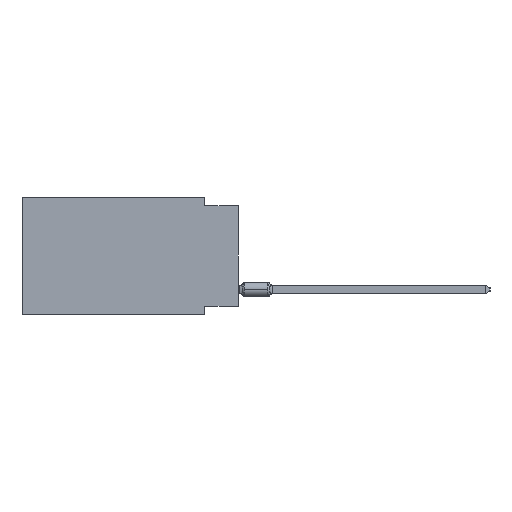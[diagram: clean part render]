
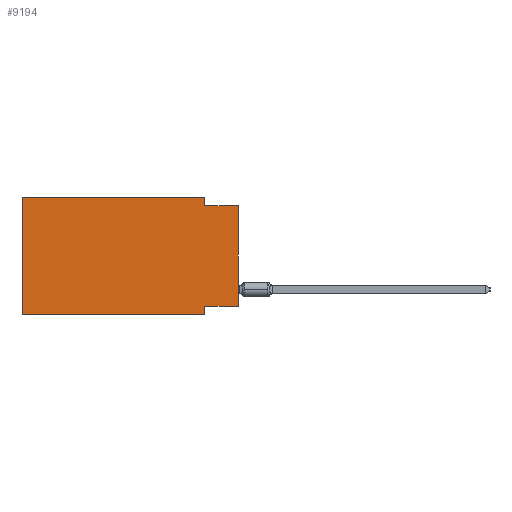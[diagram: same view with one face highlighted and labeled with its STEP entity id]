
A CAD part, left-side view. The second image highlights one B-rep face of the part: STEP entity #9194.
In plain terms, the highlighted planar face has unit normal (-1, 0, 0).
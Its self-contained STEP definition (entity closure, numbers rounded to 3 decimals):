
#537 = VECTOR ( 'NONE', #51391, 1000. ) ;
#1285 = VERTEX_POINT ( 'NONE', #85325 ) ;
#2928 = CARTESIAN_POINT ( 'NONE',  ( 0., 0., -8.255 ) ) ;
#6859 = AXIS2_PLACEMENT_3D ( 'NONE', #94778, #87290, #53614 ) ;
#9181 = ORIENTED_EDGE ( 'NONE', *, *, #14016, .T. ) ;
#9194 = ADVANCED_FACE ( 'NONE', ( #70192 ), #13004, .F. ) ;
#10488 = ORIENTED_EDGE ( 'NONE', *, *, #67953, .F. ) ;
#12084 = EDGE_CURVE ( 'NONE', #79813, #86254, #32679, .T. ) ;
#13004 = PLANE ( 'NONE',  #6859 ) ;
#14016 = EDGE_CURVE ( 'NONE', #24694, #28024, #19779, .T. ) ;
#16752 = EDGE_CURVE ( 'NONE', #86254, #28024, #59409, .T. ) ;
#16832 = EDGE_CURVE ( 'NONE', #98112, #1285, #22330, .T. ) ;
#16952 = EDGE_LOOP ( 'NONE', ( #55615, #24798, #31370, #48739, #10488, #9181, #80928, #34785 ) ) ;
#19779 = LINE ( 'NONE', #93534, #32743 ) ;
#20227 = LINE ( 'NONE', #103587, #83513 ) ;
#20298 = DIRECTION ( 'NONE',  ( 0., -1., 0. ) ) ;
#22330 = LINE ( 'NONE', #70986, #87609 ) ;
#23710 = LINE ( 'NONE', #56316, #55400 ) ;
#24694 = VERTEX_POINT ( 'NONE', #85943 ) ;
#24798 = ORIENTED_EDGE ( 'NONE', *, *, #37256, .F. ) ;
#28024 = VERTEX_POINT ( 'NONE', #82637 ) ;
#29322 = VECTOR ( 'NONE', #35909, 1000. ) ;
#31370 = ORIENTED_EDGE ( 'NONE', *, *, #16832, .F. ) ;
#32679 = LINE ( 'NONE', #81328, #54662 ) ;
#32743 = VECTOR ( 'NONE', #20298, 1000. ) ;
#34785 = ORIENTED_EDGE ( 'NONE', *, *, #12084, .F. ) ;
#35909 = DIRECTION ( 'NONE',  ( 0., 0., 1. ) ) ;
#37256 = EDGE_CURVE ( 'NONE', #1285, #48878, #42609, .T. ) ;
#40240 = CARTESIAN_POINT ( 'NONE',  ( 0., 0., -0.635 ) ) ;
#42609 = LINE ( 'NONE', #93373, #63738 ) ;
#45849 = DIRECTION ( 'NONE',  ( 0., 0., -1. ) ) ;
#48739 = ORIENTED_EDGE ( 'NONE', *, *, #76169, .F. ) ;
#48878 = VERTEX_POINT ( 'NONE', #40240 ) ;
#50125 = DIRECTION ( 'NONE',  ( 0., -1., 0. ) ) ;
#50859 = CARTESIAN_POINT ( 'NONE',  ( 0., 2.54, -8.89 ) ) ;
#51391 = DIRECTION ( 'NONE',  ( 0., 0., -1. ) ) ;
#52838 = DIRECTION ( 'NONE',  ( 0., 0., 1. ) ) ;
#53507 = LINE ( 'NONE', #60479, #29322 ) ;
#53614 = DIRECTION ( 'NONE',  ( 0., 0., -1. ) ) ;
#54662 = VECTOR ( 'NONE', #88832, 1000. ) ;
#55400 = VECTOR ( 'NONE', #88932, 1000. ) ;
#55615 = ORIENTED_EDGE ( 'NONE', *, *, #65486, .T. ) ;
#56316 = CARTESIAN_POINT ( 'NONE',  ( 0., 16.383, 0. ) ) ;
#59409 = LINE ( 'NONE', #50859, #537 ) ;
#60479 = CARTESIAN_POINT ( 'NONE',  ( 0., 16.383, 0. ) ) ;
#63738 = VECTOR ( 'NONE', #50125, 1000. ) ;
#65486 = EDGE_CURVE ( 'NONE', #79813, #48878, #20227, .T. ) ;
#65684 = CARTESIAN_POINT ( 'NONE',  ( 0., 2.54, 0. ) ) ;
#67592 = CARTESIAN_POINT ( 'NONE',  ( 0., 16.383, 0. ) ) ;
#67953 = EDGE_CURVE ( 'NONE', #24694, #102076, #53507, .T. ) ;
#70192 = FACE_OUTER_BOUND ( 'NONE', #16952, .T. ) ;
#70986 = CARTESIAN_POINT ( 'NONE',  ( 0., 2.54, 0. ) ) ;
#76169 = EDGE_CURVE ( 'NONE', #102076, #98112, #23710, .T. ) ;
#79813 = VERTEX_POINT ( 'NONE', #2928 ) ;
#80928 = ORIENTED_EDGE ( 'NONE', *, *, #16752, .F. ) ;
#81328 = CARTESIAN_POINT ( 'NONE',  ( 0., 0., -8.255 ) ) ;
#82637 = CARTESIAN_POINT ( 'NONE',  ( 0., 2.54, -8.89 ) ) ;
#83513 = VECTOR ( 'NONE', #52838, 1000. ) ;
#85325 = CARTESIAN_POINT ( 'NONE',  ( 0., 2.54, -0.635 ) ) ;
#85943 = CARTESIAN_POINT ( 'NONE',  ( 0., 16.383, -8.89 ) ) ;
#86254 = VERTEX_POINT ( 'NONE', #90150 ) ;
#87290 = DIRECTION ( 'NONE',  ( 1., 0., 0. ) ) ;
#87609 = VECTOR ( 'NONE', #45849, 1000. ) ;
#88832 = DIRECTION ( 'NONE',  ( 0., 1., 0. ) ) ;
#88932 = DIRECTION ( 'NONE',  ( 0., -1., 0. ) ) ;
#90150 = CARTESIAN_POINT ( 'NONE',  ( 0., 2.54, -8.255 ) ) ;
#93373 = CARTESIAN_POINT ( 'NONE',  ( 0., 0., -0.635 ) ) ;
#93534 = CARTESIAN_POINT ( 'NONE',  ( 0., 16.383, -8.89 ) ) ;
#94778 = CARTESIAN_POINT ( 'NONE',  ( 0., 16.383, 0. ) ) ;
#98112 = VERTEX_POINT ( 'NONE', #65684 ) ;
#102076 = VERTEX_POINT ( 'NONE', #67592 ) ;
#103587 = CARTESIAN_POINT ( 'NONE',  ( 0., 0., 0. ) ) ;
